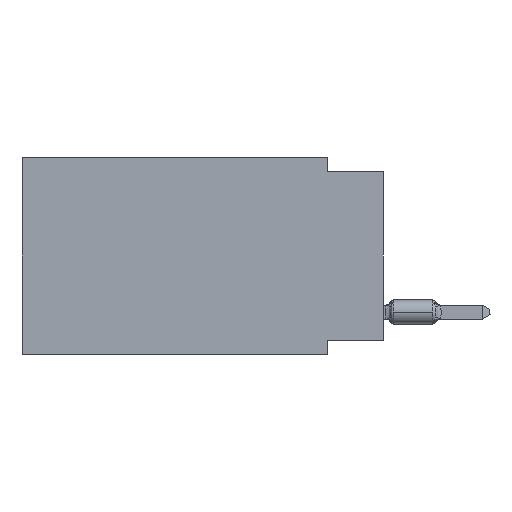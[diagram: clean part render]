
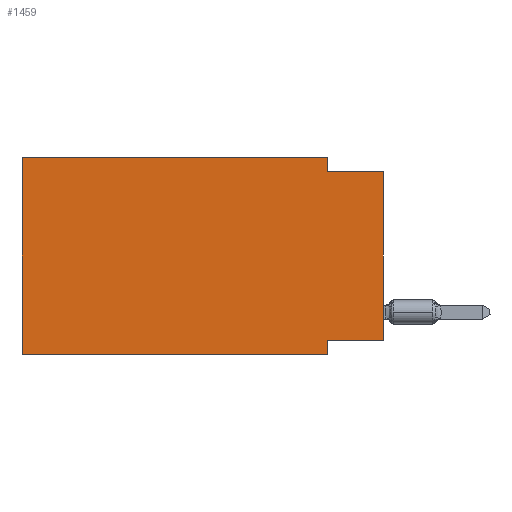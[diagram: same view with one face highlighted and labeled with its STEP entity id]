
A CAD part, left-side view. The second image highlights one B-rep face of the part: STEP entity #1459.
In plain terms, the highlighted planar face has unit normal (-1, 0, 0).
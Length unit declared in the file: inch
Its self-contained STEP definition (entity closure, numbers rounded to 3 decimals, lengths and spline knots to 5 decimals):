
#636 = VERTEX_POINT ( 'NONE', #8547 ) ;
#1173 = CARTESIAN_POINT ( 'NONE',  ( 0., 0.1, -0.025 ) ) ;
#1459 = ADVANCED_FACE ( 'NONE', ( #13820 ), #41437, .F. ) ;
#1695 = EDGE_CURVE ( 'NONE', #25223, #13270, #34513, .T. ) ;
#2964 = DIRECTION ( 'NONE',  ( 0., -1., 0. ) ) ;
#3449 = DIRECTION ( 'NONE',  ( 0., 1., 0. ) ) ;
#4134 = EDGE_CURVE ( 'NONE', #49462, #32277, #24293, .T. ) ;
#5373 = CARTESIAN_POINT ( 'NONE',  ( 0., 0.645, -0.35 ) ) ;
#5592 = ORIENTED_EDGE ( 'NONE', *, *, #21999, .F. ) ;
#7246 = CARTESIAN_POINT ( 'NONE',  ( 0., 0.645, -0.35 ) ) ;
#7885 = EDGE_CURVE ( 'NONE', #48182, #26683, #22400, .T. ) ;
#7961 = VECTOR ( 'NONE', #9225, 39.37008 ) ;
#8547 = CARTESIAN_POINT ( 'NONE',  ( 0., 0.1, -0.325 ) ) ;
#9225 = DIRECTION ( 'NONE',  ( 0., -1., 0. ) ) ;
#9588 = LINE ( 'NONE', #12704, #19944 ) ;
#9882 = EDGE_LOOP ( 'NONE', ( #24869, #26563, #28526, #9998, #5592, #39639, #43627, #23145 ) ) ;
#9998 = ORIENTED_EDGE ( 'NONE', *, *, #7885, .F. ) ;
#10239 = AXIS2_PLACEMENT_3D ( 'NONE', #33019, #44764, #36836 ) ;
#10310 = CARTESIAN_POINT ( 'NONE',  ( 0., 0.1, -0.35 ) ) ;
#10327 = CARTESIAN_POINT ( 'NONE',  ( 0., 0.645, 0. ) ) ;
#12180 = CARTESIAN_POINT ( 'NONE',  ( 0., 0., -0.325 ) ) ;
#12704 = CARTESIAN_POINT ( 'NONE',  ( 0., 0.645, 0. ) ) ;
#13270 = VERTEX_POINT ( 'NONE', #41454 ) ;
#13745 = DIRECTION ( 'NONE',  ( 0., 0., 1. ) ) ;
#13820 = FACE_OUTER_BOUND ( 'NONE', #9882, .T. ) ;
#15084 = DIRECTION ( 'NONE',  ( 0., -1., 0. ) ) ;
#15227 = DIRECTION ( 'NONE',  ( 0., 0., -1. ) ) ;
#18310 = LINE ( 'NONE', #33898, #25131 ) ;
#19676 = CARTESIAN_POINT ( 'NONE',  ( 0., 0., -0.025 ) ) ;
#19944 = VECTOR ( 'NONE', #47967, 39.37008 ) ;
#21704 = CARTESIAN_POINT ( 'NONE',  ( 0., 0.1, -0.35 ) ) ;
#21999 = EDGE_CURVE ( 'NONE', #49462, #48182, #9588, .T. ) ;
#22400 = LINE ( 'NONE', #38011, #47372 ) ;
#23145 = ORIENTED_EDGE ( 'NONE', *, *, #30008, .F. ) ;
#24293 = LINE ( 'NONE', #5373, #7961 ) ;
#24869 = ORIENTED_EDGE ( 'NONE', *, *, #25051, .T. ) ;
#24898 = VECTOR ( 'NONE', #25887, 39.37008 ) ;
#25051 = EDGE_CURVE ( 'NONE', #25141, #13270, #38268, .T. ) ;
#25131 = VECTOR ( 'NONE', #15227, 39.37008 ) ;
#25141 = VERTEX_POINT ( 'NONE', #12180 ) ;
#25223 = VERTEX_POINT ( 'NONE', #1173 ) ;
#25887 = DIRECTION ( 'NONE',  ( 0., 0., -1. ) ) ;
#26563 = ORIENTED_EDGE ( 'NONE', *, *, #1695, .F. ) ;
#26683 = VERTEX_POINT ( 'NONE', #36443 ) ;
#28526 = ORIENTED_EDGE ( 'NONE', *, *, #35739, .F. ) ;
#30008 = EDGE_CURVE ( 'NONE', #25141, #636, #30803, .T. ) ;
#30803 = LINE ( 'NONE', #42094, #32568 ) ;
#32277 = VERTEX_POINT ( 'NONE', #21704 ) ;
#32568 = VECTOR ( 'NONE', #3449, 39.37008 ) ;
#33019 = CARTESIAN_POINT ( 'NONE',  ( 0., 0.645, 0. ) ) ;
#33840 = LINE ( 'NONE', #10310, #24898 ) ;
#33898 = CARTESIAN_POINT ( 'NONE',  ( 0., 0.1, 0. ) ) ;
#34513 = LINE ( 'NONE', #19676, #45267 ) ;
#35739 = EDGE_CURVE ( 'NONE', #26683, #25223, #18310, .T. ) ;
#36443 = CARTESIAN_POINT ( 'NONE',  ( 0., 0.1, 0. ) ) ;
#36836 = DIRECTION ( 'NONE',  ( 0., 0., -1. ) ) ;
#38011 = CARTESIAN_POINT ( 'NONE',  ( 0., 0.645, 0. ) ) ;
#38268 = LINE ( 'NONE', #48770, #48893 ) ;
#39639 = ORIENTED_EDGE ( 'NONE', *, *, #4134, .T. ) ;
#41437 = PLANE ( 'NONE',  #10239 ) ;
#41454 = CARTESIAN_POINT ( 'NONE',  ( 0., 0., -0.025 ) ) ;
#42094 = CARTESIAN_POINT ( 'NONE',  ( 0., 0., -0.325 ) ) ;
#43627 = ORIENTED_EDGE ( 'NONE', *, *, #45634, .F. ) ;
#44764 = DIRECTION ( 'NONE',  ( 1., 0., 0. ) ) ;
#45267 = VECTOR ( 'NONE', #15084, 39.37008 ) ;
#45634 = EDGE_CURVE ( 'NONE', #636, #32277, #33840, .T. ) ;
#47372 = VECTOR ( 'NONE', #2964, 39.37008 ) ;
#47967 = DIRECTION ( 'NONE',  ( 0., 0., 1. ) ) ;
#48182 = VERTEX_POINT ( 'NONE', #10327 ) ;
#48770 = CARTESIAN_POINT ( 'NONE',  ( 0., 0., 0. ) ) ;
#48893 = VECTOR ( 'NONE', #13745, 39.37008 ) ;
#49462 = VERTEX_POINT ( 'NONE', #7246 ) ;
